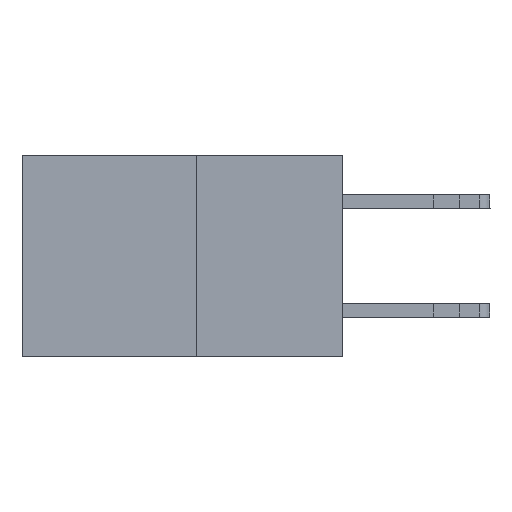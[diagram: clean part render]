
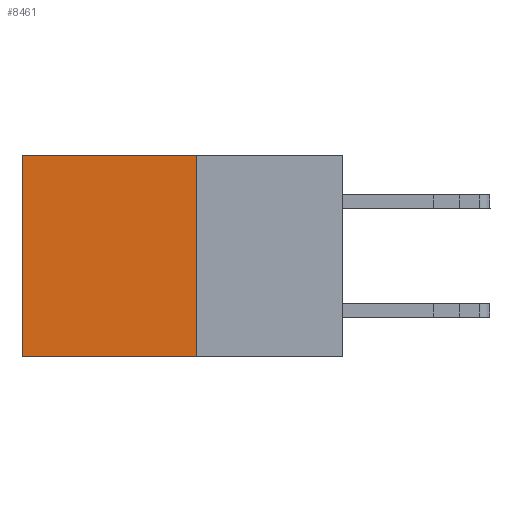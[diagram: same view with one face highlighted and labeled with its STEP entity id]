
A CAD part, left-side view. The second image highlights one B-rep face of the part: STEP entity #8461.
In plain terms, the highlighted planar face has unit normal (-1, 0, 0).
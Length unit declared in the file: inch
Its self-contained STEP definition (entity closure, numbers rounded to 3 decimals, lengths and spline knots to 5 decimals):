
#1460 = LINE ( 'NONE', #14257, #5546 ) ;
#1959 = CARTESIAN_POINT ( 'NONE',  ( 0.277, 0.27, 0. ) ) ;
#2787 = VECTOR ( 'NONE', #10542, 39.37008 ) ;
#3387 = EDGE_CURVE ( 'NONE', #16785, #9799, #6410, .T. ) ;
#4137 = CARTESIAN_POINT ( 'NONE',  ( 0.277, 0.59, -0.37 ) ) ;
#4233 = CARTESIAN_POINT ( 'NONE',  ( 0.277, 0.27, -0.37 ) ) ;
#4692 = CARTESIAN_POINT ( 'NONE',  ( 0.277, 0.27, 0. ) ) ;
#5222 = FACE_OUTER_BOUND ( 'NONE', #18164, .T. ) ;
#5546 = VECTOR ( 'NONE', #6704, 39.37008 ) ;
#5646 = VERTEX_POINT ( 'NONE', #4137 ) ;
#6351 = VECTOR ( 'NONE', #11515, 39.37008 ) ;
#6410 = LINE ( 'NONE', #1959, #18043 ) ;
#6704 = DIRECTION ( 'NONE',  ( 0., 0., -1. ) ) ;
#7171 = CARTESIAN_POINT ( 'NONE',  ( 0.277, 0.27, -0.37 ) ) ;
#8461 = ADVANCED_FACE ( 'NONE', ( #5222 ), #17758, .F. ) ;
#9618 = DIRECTION ( 'NONE',  ( 0., 1., 0. ) ) ;
#9799 = VERTEX_POINT ( 'NONE', #10646 ) ;
#10012 = CARTESIAN_POINT ( 'NONE',  ( 0.277, 0.27, -0.37 ) ) ;
#10261 = DIRECTION ( 'NONE',  ( 0., 0., -1. ) ) ;
#10542 = DIRECTION ( 'NONE',  ( 0., 0., -1. ) ) ;
#10646 = CARTESIAN_POINT ( 'NONE',  ( 0.277, 0.59, 0. ) ) ;
#10830 = EDGE_CURVE ( 'NONE', #16578, #5646, #14403, .T. ) ;
#10930 = LINE ( 'NONE', #13467, #2787 ) ;
#11077 = EDGE_CURVE ( 'NONE', #9799, #5646, #10930, .T. ) ;
#11515 = DIRECTION ( 'NONE',  ( 0., 1., 0. ) ) ;
#13467 = CARTESIAN_POINT ( 'NONE',  ( 0.277, 0.59, -0.37 ) ) ;
#14257 = CARTESIAN_POINT ( 'NONE',  ( 0.277, 0.27, -0.37 ) ) ;
#14403 = LINE ( 'NONE', #10012, #6351 ) ;
#14658 = EDGE_CURVE ( 'NONE', #16785, #16578, #1460, .T. ) ;
#14664 = ORIENTED_EDGE ( 'NONE', *, *, #14658, .F. ) ;
#15366 = ORIENTED_EDGE ( 'NONE', *, *, #11077, .T. ) ;
#16578 = VERTEX_POINT ( 'NONE', #4233 ) ;
#16785 = VERTEX_POINT ( 'NONE', #4692 ) ;
#17302 = ORIENTED_EDGE ( 'NONE', *, *, #10830, .F. ) ;
#17389 = AXIS2_PLACEMENT_3D ( 'NONE', #7171, #19257, #10261 ) ;
#17758 = PLANE ( 'NONE',  #17389 ) ;
#18043 = VECTOR ( 'NONE', #9618, 39.37008 ) ;
#18164 = EDGE_LOOP ( 'NONE', ( #15366, #17302, #14664, #18710 ) ) ;
#18710 = ORIENTED_EDGE ( 'NONE', *, *, #3387, .T. ) ;
#19257 = DIRECTION ( 'NONE',  ( 1., 0., 0. ) ) ;
